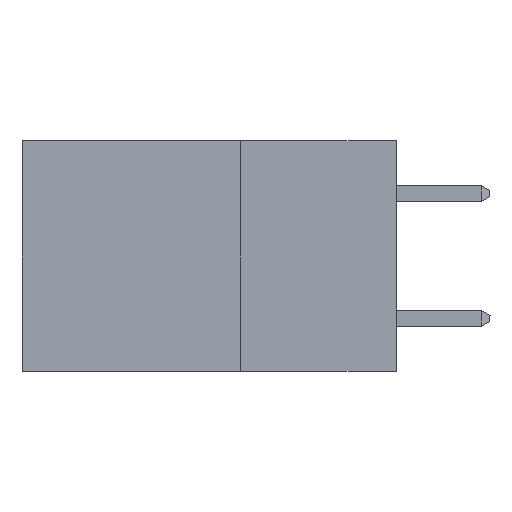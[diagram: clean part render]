
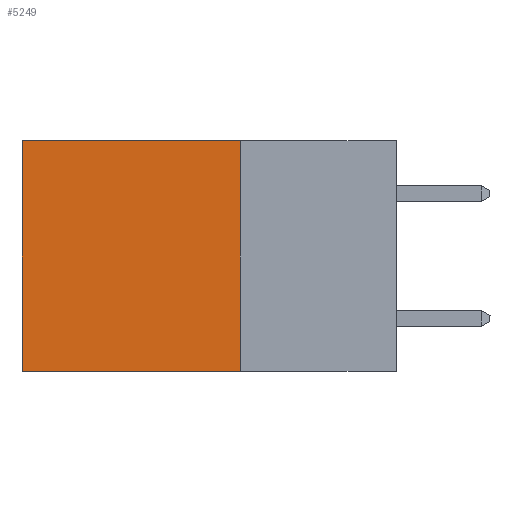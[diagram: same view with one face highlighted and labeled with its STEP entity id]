
A CAD part, left-side view. The second image highlights one B-rep face of the part: STEP entity #5249.
In plain terms, the highlighted planar face has unit normal (-1, 0, 0).
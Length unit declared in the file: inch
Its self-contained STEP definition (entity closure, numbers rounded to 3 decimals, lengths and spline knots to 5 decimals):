
#577 = ORIENTED_EDGE ( 'NONE', *, *, #6643, .T. ) ;
#1662 = ORIENTED_EDGE ( 'NONE', *, *, #10587, .F. ) ;
#2242 = VERTEX_POINT ( 'NONE', #6809 ) ;
#2405 = FACE_OUTER_BOUND ( 'NONE', #4450, .T. ) ;
#3056 = ORIENTED_EDGE ( 'NONE', *, *, #8202, .T. ) ;
#3455 = DIRECTION ( 'NONE',  ( 0., 1., 0. ) ) ;
#3700 = VECTOR ( 'NONE', #10428, 39.37008 ) ;
#3752 = CARTESIAN_POINT ( 'NONE',  ( 0.2615, 0.25, -0.37 ) ) ;
#4187 = EDGE_CURVE ( 'NONE', #11519, #11264, #11711, .T. ) ;
#4450 = EDGE_LOOP ( 'NONE', ( #577, #1662, #6137, #3056 ) ) ;
#5249 = ADVANCED_FACE ( 'NONE', ( #2405 ), #7582, .F. ) ;
#5598 = CARTESIAN_POINT ( 'NONE',  ( 0.2615, 0.6, -0.37 ) ) ;
#5988 = VECTOR ( 'NONE', #8732, 39.37008 ) ;
#6137 = ORIENTED_EDGE ( 'NONE', *, *, #4187, .F. ) ;
#6643 = EDGE_CURVE ( 'NONE', #2242, #9197, #11487, .T. ) ;
#6809 = CARTESIAN_POINT ( 'NONE',  ( 0.2615, 0.6, 0. ) ) ;
#7498 = DIRECTION ( 'NONE',  ( 0., 0., -1. ) ) ;
#7544 = DIRECTION ( 'NONE',  ( 1., 0., 0. ) ) ;
#7582 = PLANE ( 'NONE',  #10570 ) ;
#7707 = CARTESIAN_POINT ( 'NONE',  ( 0.2615, 0.25, -0.37 ) ) ;
#8202 = EDGE_CURVE ( 'NONE', #11519, #2242, #10052, .T. ) ;
#8732 = DIRECTION ( 'NONE',  ( 0., 0., -1. ) ) ;
#8900 = CARTESIAN_POINT ( 'NONE',  ( 0.2615, 0.25, 0. ) ) ;
#9197 = VERTEX_POINT ( 'NONE', #5598 ) ;
#9260 = CARTESIAN_POINT ( 'NONE',  ( 0.2615, 0.6, -0.37 ) ) ;
#10052 = LINE ( 'NONE', #11219, #12999 ) ;
#10386 = VECTOR ( 'NONE', #3455, 39.37008 ) ;
#10413 = CARTESIAN_POINT ( 'NONE',  ( 0.2615, 0.25, -0.37 ) ) ;
#10428 = DIRECTION ( 'NONE',  ( 0., 0., -1. ) ) ;
#10570 = AXIS2_PLACEMENT_3D ( 'NONE', #7707, #7544, #7498 ) ;
#10587 = EDGE_CURVE ( 'NONE', #11264, #9197, #13028, .T. ) ;
#10803 = CARTESIAN_POINT ( 'NONE',  ( 0.2615, 0.25, -0.37 ) ) ;
#11204 = DIRECTION ( 'NONE',  ( 0., 1., 0. ) ) ;
#11219 = CARTESIAN_POINT ( 'NONE',  ( 0.2615, 0.25, 0. ) ) ;
#11264 = VERTEX_POINT ( 'NONE', #10803 ) ;
#11487 = LINE ( 'NONE', #9260, #5988 ) ;
#11519 = VERTEX_POINT ( 'NONE', #8900 ) ;
#11711 = LINE ( 'NONE', #10413, #3700 ) ;
#12999 = VECTOR ( 'NONE', #11204, 39.37008 ) ;
#13028 = LINE ( 'NONE', #3752, #10386 ) ;
